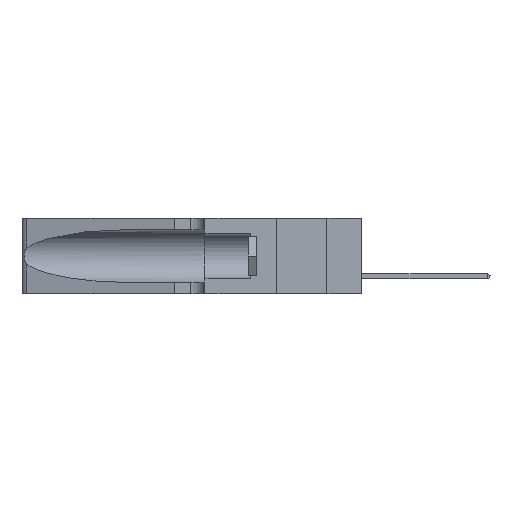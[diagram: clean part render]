
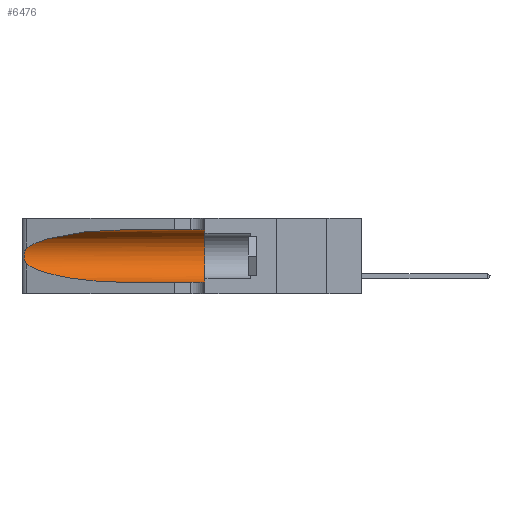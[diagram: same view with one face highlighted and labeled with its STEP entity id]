
A CAD part, left-side view. The second image highlights one B-rep face of the part: STEP entity #6476.
In plain terms, the highlighted cylindrical face has radius 3.308 mm (diameter 6.617 mm), a partial arc.
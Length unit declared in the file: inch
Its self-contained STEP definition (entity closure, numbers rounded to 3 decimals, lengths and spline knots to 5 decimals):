
#389 = CARTESIAN_POINT ( 'NONE',  ( 0.1305, 0.35, 0.05475 ) ) ;
#427 = CARTESIAN_POINT ( 'NONE',  ( 0.18966, 0.96281, 0.05475 ) ) ;
#620 = EDGE_CURVE ( 'NONE', #28083, #7125, #14349, .T. ) ;
#740 = EDGE_CURVE ( 'NONE', #12739, #7125, #28714, .T. ) ;
#751 = FACE_OUTER_BOUND ( 'NONE', #16456, .T. ) ;
#2217 = CARTESIAN_POINT ( 'NONE',  ( 0.25487, 1.22718, 0.22369 ) ) ;
#4357 = CARTESIAN_POINT ( 'NONE',  ( 0.25555, 1.22994, 0.2215 ) ) ;
#4417 = CARTESIAN_POINT ( 'NONE',  ( 0.26017, 1.23833, 0.17102 ) ) ;
#4490 = CARTESIAN_POINT ( 'NONE',  ( 0.25487, 1.22718, 0.14631 ) ) ;
#4606 = CARTESIAN_POINT ( 'NONE',  ( 0.25789, 1.23486, 0.15765 ) ) ;
#5119 = EDGE_CURVE ( 'NONE', #21351, #8123, #27777, .T. ) ;
#5757 = CARTESIAN_POINT ( 'NONE',  ( 0.1305, 0.35, 0.185 ) ) ;
#5995 = ORIENTED_EDGE ( 'NONE', *, *, #740, .T. ) ;
#6476 = ADVANCED_FACE ( 'NONE', ( #751 ), #21088, .F. ) ;
#7125 = VERTEX_POINT ( 'NONE', #389 ) ;
#7175 = CARTESIAN_POINT ( 'NONE',  ( 0.25487, 1.22718, 0.14631 ) ) ;
#8123 = VERTEX_POINT ( 'NONE', #11272 ) ;
#8410 =( BOUNDED_CURVE ( )  B_SPLINE_CURVE ( 3, ( #19000, #10280, #17209, #11187 ),
 .UNSPECIFIED., .F., .F. ) 
 B_SPLINE_CURVE_WITH_KNOTS ( ( 4, 4 ),
 ( 1.5708, 2.84003 ),
 .UNSPECIFIED. ) 
 CURVE ( )  GEOMETRIC_REPRESENTATION_ITEM ( )  RATIONAL_B_SPLINE_CURVE ( ( 1., 0.87, 0.87, 1. ) ) 
 REPRESENTATION_ITEM ( '' )  );
#8570 = CARTESIAN_POINT ( 'NONE',  ( 0.25487, 1.22718, 0.22369 ) ) ;
#9029 = AXIS2_PLACEMENT_3D ( 'NONE', #22750, #20327, #27309 ) ;
#9254 = LINE ( 'NONE', #23161, #17366 ) ;
#9535 = ORIENTED_EDGE ( 'NONE', *, *, #15355, .T. ) ;
#10280 = CARTESIAN_POINT ( 'NONE',  ( 0.18966, 0.96281, 0.31525 ) ) ;
#10840 = DIRECTION ( 'NONE',  ( 0., 0., 1. ) ) ;
#10996 = CARTESIAN_POINT ( 'NONE',  ( 0.1305, 1.61858, 0.05475 ) ) ;
#11187 = CARTESIAN_POINT ( 'NONE',  ( 0.25487, 1.22718, 0.22369 ) ) ;
#11272 = CARTESIAN_POINT ( 'NONE',  ( 0.25487, 1.22718, 0.14631 ) ) ;
#11337 = CARTESIAN_POINT ( 'NONE',  ( 0.25639, 1.23186, 0.15144 ) ) ;
#11349 = CARTESIAN_POINT ( 'NONE',  ( 0.1305, 0.72297, 0.05475 ) ) ;
#11667 = DIRECTION ( 'NONE',  ( 0., -1., 0. ) ) ;
#12739 = VERTEX_POINT ( 'NONE', #14463 ) ;
#13407 = CARTESIAN_POINT ( 'NONE',  ( 0.25856, 1.23593, 0.16098 ) ) ;
#13577 =( BOUNDED_CURVE ( )  B_SPLINE_CURVE ( 3, ( #7175, #27213, #427, #11349 ),
 .UNSPECIFIED., .F., .F. ) 
 B_SPLINE_CURVE_WITH_KNOTS ( ( 4, 4 ),
 ( 3.44316, 4.71239 ),
 .UNSPECIFIED. ) 
 CURVE ( )  GEOMETRIC_REPRESENTATION_ITEM ( )  RATIONAL_B_SPLINE_CURVE ( ( 1., 0.87, 0.87, 1. ) ) 
 REPRESENTATION_ITEM ( '' )  );
#13588 = CARTESIAN_POINT ( 'NONE',  ( 0.26075, 1.23896, 0.19203 ) ) ;
#14349 = CIRCLE ( 'NONE', #22266, 0.13025 ) ;
#14463 = CARTESIAN_POINT ( 'NONE',  ( 0.1305, 0.72297, 0.05475 ) ) ;
#15355 = EDGE_CURVE ( 'NONE', #20594, #21351, #8410, .T. ) ;
#16456 = EDGE_LOOP ( 'NONE', ( #9535, #22022, #20504, #5995, #19948, #18786 ) ) ;
#16484 = EDGE_CURVE ( 'NONE', #8123, #12739, #13577, .T. ) ;
#17209 = CARTESIAN_POINT ( 'NONE',  ( 0.2373, 1.15595, 0.28018 ) ) ;
#17366 = VECTOR ( 'NONE', #21126, 39.37008 ) ;
#17854 = CARTESIAN_POINT ( 'NONE',  ( 0.26075, 1.23896, 0.178 ) ) ;
#18786 = ORIENTED_EDGE ( 'NONE', *, *, #27639, .F. ) ;
#19000 = CARTESIAN_POINT ( 'NONE',  ( 0.1305, 0.72297, 0.31525 ) ) ;
#19295 = CARTESIAN_POINT ( 'NONE',  ( 0.25854, 1.2359, 0.20912 ) ) ;
#19641 = CARTESIAN_POINT ( 'NONE',  ( 0.25639, 1.23184, 0.21858 ) ) ;
#19948 = ORIENTED_EDGE ( 'NONE', *, *, #620, .F. ) ;
#20327 = DIRECTION ( 'NONE',  ( 0., -1., 0. ) ) ;
#20504 = ORIENTED_EDGE ( 'NONE', *, *, #16484, .T. ) ;
#20594 = VERTEX_POINT ( 'NONE', #22132 ) ;
#21088 = CYLINDRICAL_SURFACE ( 'NONE', #9029, 0.13025 ) ;
#21126 = DIRECTION ( 'NONE',  ( 0., -1., 0. ) ) ;
#21344 = CARTESIAN_POINT ( 'NONE',  ( 0.25787, 1.23484, 0.2124 ) ) ;
#21351 = VERTEX_POINT ( 'NONE', #2217 ) ;
#21752 = VECTOR ( 'NONE', #11667, 39.37008 ) ;
#22022 = ORIENTED_EDGE ( 'NONE', *, *, #5119, .T. ) ;
#22132 = CARTESIAN_POINT ( 'NONE',  ( 0.1305, 0.72297, 0.31525 ) ) ;
#22266 = AXIS2_PLACEMENT_3D ( 'NONE', #5757, #23708, #10840 ) ;
#22750 = CARTESIAN_POINT ( 'NONE',  ( 0.1305, 1.61858, 0.185 ) ) ;
#23161 = CARTESIAN_POINT ( 'NONE',  ( 0.1305, 1.61858, 0.31525 ) ) ;
#23708 = DIRECTION ( 'NONE',  ( 0., 1., 0. ) ) ;
#24870 = CARTESIAN_POINT ( 'NONE',  ( 0.26018, 1.23835, 0.19895 ) ) ;
#26995 = CARTESIAN_POINT ( 'NONE',  ( 0.25555, 1.22993, 0.14849 ) ) ;
#27213 = CARTESIAN_POINT ( 'NONE',  ( 0.2373, 1.15595, 0.08982 ) ) ;
#27309 = DIRECTION ( 'NONE',  ( 0., 0., -1. ) ) ;
#27639 = EDGE_CURVE ( 'NONE', #20594, #28083, #9254, .T. ) ;
#27777 = B_SPLINE_CURVE_WITH_KNOTS ( 'NONE', 3,
 ( #8570, #4357, #19641, #21344, #19295, #24870, #13588, #17854, #4417, #13407, #4606, #11337, #26995, #4490 ),
 .UNSPECIFIED., .F., .F.,
 ( 4, 2, 2, 2, 2, 2, 4 ),
 ( 0., 0.00027, 0.00053, 0.00107, 0.0016, 0.00187, 0.00214 ),
 .UNSPECIFIED. ) ;
#27884 = CARTESIAN_POINT ( 'NONE',  ( 0.1305, 0.35, 0.31525 ) ) ;
#28083 = VERTEX_POINT ( 'NONE', #27884 ) ;
#28714 = LINE ( 'NONE', #10996, #21752 ) ;
